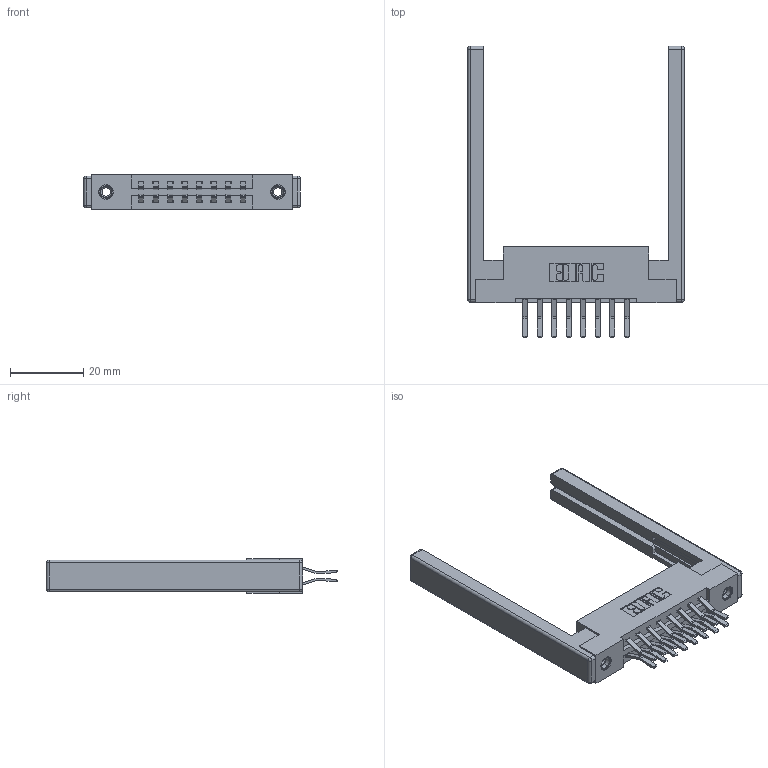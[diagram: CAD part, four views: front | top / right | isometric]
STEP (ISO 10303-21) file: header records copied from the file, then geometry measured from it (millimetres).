
FILE_DESCRIPTION (( 'STEP AP203' ), '1' );
FILE_NAME ('337-016-560-268.STEP', '2019-10-08T12:51:43', ( '' ), ( '' ), 'SwSTEP 2.0', 'SolidWorks 2016', '' );
FILE_SCHEMA (( 'CONFIG_CONTROL_DESIGN' ));
Length unit declared in the file: inch
Products named in the file (5): 345-250-001_345-250-001-102; 345-292-001_560 Tail; 307-220-068; 337-016-560-268; 337 Part_Flush Mounting Lugs - 0.156 Dia-TI
Assembly tree (21 placements, depth 2):
  337-016-560-268
    337 Part_Flush Mounting Lugs - 0.156 Dia-TI
    345-292-001_560 Tail  x16
    345-250-001_345-250-001-102  x2
    307-220-068  x2
Bounding box: 59.13 x 79.52 x 9.4 mm (x, y, z)
Volume: 10268.8 mm3; surface area: 10659.5 mm2
Topology: 21 solids, 21 shells, 1164 faces, 3373 edges, 2206 vertices
Faces by surface type: plane 766, cylinder 374, cone 12, sphere 8, torus 4
Entity records: 13448 total; most frequent: CARTESIAN_POINT 2259, ORIENTED_EDGE 2184, DIRECTION 2058, EDGE_CURVE 1092, LINE 910, VECTOR 910, VERTEX_POINT 718, AXIS2_PLACEMENT_3D 574
